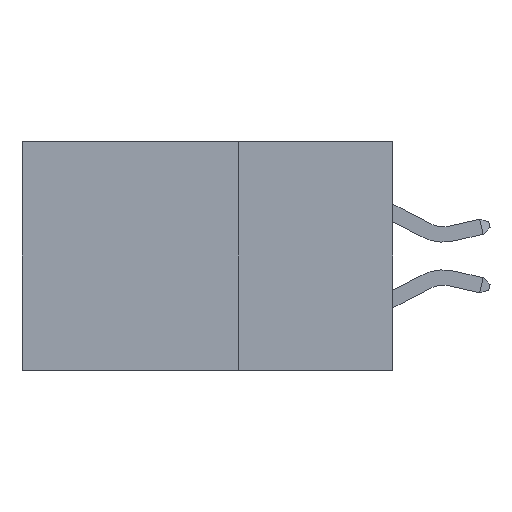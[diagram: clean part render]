
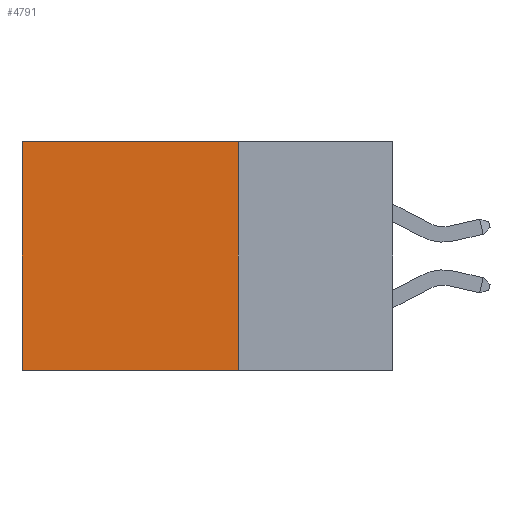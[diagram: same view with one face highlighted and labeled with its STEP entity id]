
A CAD part, left-side view. The second image highlights one B-rep face of the part: STEP entity #4791.
In plain terms, the highlighted planar face has unit normal (-1, 0, 0).
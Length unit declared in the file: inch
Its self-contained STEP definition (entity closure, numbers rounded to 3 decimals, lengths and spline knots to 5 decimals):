
#75 = LINE ( 'NONE', #14440, #12695 ) ;
#488 = VERTEX_POINT ( 'NONE', #5104 ) ;
#543 = DIRECTION ( 'NONE',  ( 0., 0., -1. ) ) ;
#1182 = VERTEX_POINT ( 'NONE', #13961 ) ;
#2798 = ORIENTED_EDGE ( 'NONE', *, *, #7456, .T. ) ;
#2842 = ORIENTED_EDGE ( 'NONE', *, *, #6275, .F. ) ;
#3646 = ORIENTED_EDGE ( 'NONE', *, *, #14675, .T. ) ;
#4791 = ADVANCED_FACE ( 'NONE', ( #8763 ), #11036, .F. ) ;
#5104 = CARTESIAN_POINT ( 'NONE',  ( 0.2875, 0.25, 0. ) ) ;
#5490 = VECTOR ( 'NONE', #543, 39.37008 ) ;
#6275 = EDGE_CURVE ( 'NONE', #488, #11846, #12331, .T. ) ;
#7450 = CARTESIAN_POINT ( 'NONE',  ( 0.2875, 0.25, -0.37 ) ) ;
#7456 = EDGE_CURVE ( 'NONE', #15268, #1182, #14474, .T. ) ;
#7999 = EDGE_LOOP ( 'NONE', ( #2798, #15309, #2842, #3646 ) ) ;
#8043 = CARTESIAN_POINT ( 'NONE',  ( 0.2875, 0.6, 0. ) ) ;
#8763 = FACE_OUTER_BOUND ( 'NONE', #7999, .T. ) ;
#9177 = DIRECTION ( 'NONE',  ( 0., 0., -1. ) ) ;
#9281 = CARTESIAN_POINT ( 'NONE',  ( 0.2875, 0.25, 0. ) ) ;
#10357 = VECTOR ( 'NONE', #10975, 39.37008 ) ;
#10707 = LINE ( 'NONE', #7450, #10357 ) ;
#10962 = DIRECTION ( 'NONE',  ( 0., 0., -1. ) ) ;
#10963 = DIRECTION ( 'NONE',  ( 0., 1., 0. ) ) ;
#10973 = DIRECTION ( 'NONE',  ( 1., 0., 0. ) ) ;
#10975 = DIRECTION ( 'NONE',  ( 0., 1., 0. ) ) ;
#11012 = CARTESIAN_POINT ( 'NONE',  ( 0.2875, 0.25, 0. ) ) ;
#11036 = PLANE ( 'NONE',  #15285 ) ;
#11281 = EDGE_CURVE ( 'NONE', #11846, #1182, #10707, .T. ) ;
#11846 = VERTEX_POINT ( 'NONE', #15419 ) ;
#12331 = LINE ( 'NONE', #9281, #15044 ) ;
#12695 = VECTOR ( 'NONE', #10963, 39.37008 ) ;
#13961 = CARTESIAN_POINT ( 'NONE',  ( 0.2875, 0.6, -0.37 ) ) ;
#14420 = CARTESIAN_POINT ( 'NONE',  ( 0.2875, 0.6, 0. ) ) ;
#14440 = CARTESIAN_POINT ( 'NONE',  ( 0.2875, 0.25, 0. ) ) ;
#14474 = LINE ( 'NONE', #8043, #5490 ) ;
#14675 = EDGE_CURVE ( 'NONE', #488, #15268, #75, .T. ) ;
#15044 = VECTOR ( 'NONE', #9177, 39.37008 ) ;
#15268 = VERTEX_POINT ( 'NONE', #14420 ) ;
#15285 = AXIS2_PLACEMENT_3D ( 'NONE', #11012, #10973, #10962 ) ;
#15309 = ORIENTED_EDGE ( 'NONE', *, *, #11281, .F. ) ;
#15419 = CARTESIAN_POINT ( 'NONE',  ( 0.2875, 0.25, -0.37 ) ) ;
